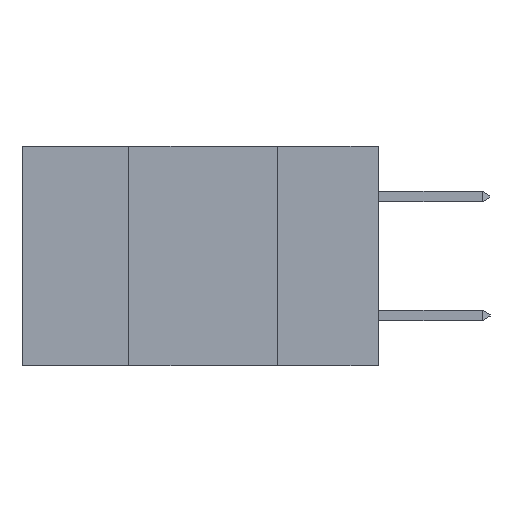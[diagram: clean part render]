
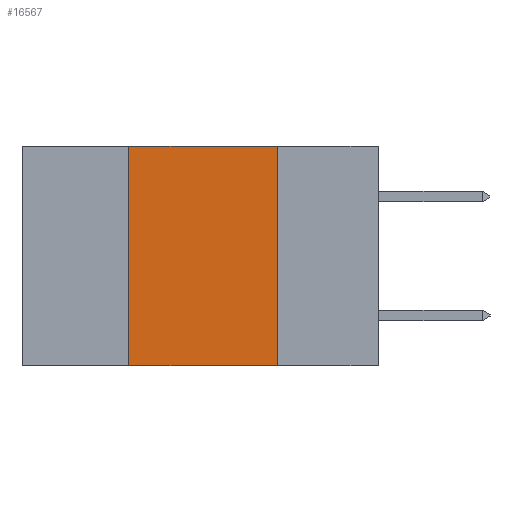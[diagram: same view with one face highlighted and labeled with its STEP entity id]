
A CAD part, left-side view. The second image highlights one B-rep face of the part: STEP entity #16567.
In plain terms, the highlighted planar face has unit normal (-1, 0, 0).
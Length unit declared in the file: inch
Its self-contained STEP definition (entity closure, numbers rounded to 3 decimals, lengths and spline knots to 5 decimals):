
#3025 = AXIS2_PLACEMENT_3D ( 'NONE', #11311, #7269, #16801 ) ;
#3606 = ORIENTED_EDGE ( 'NONE', *, *, #10193, .F. ) ;
#3710 = VERTEX_POINT ( 'NONE', #5674 ) ;
#4558 = ORIENTED_EDGE ( 'NONE', *, *, #13758, .F. ) ;
#4705 = VECTOR ( 'NONE', #7271, 39.37008 ) ;
#5646 = ORIENTED_EDGE ( 'NONE', *, *, #12043, .F. ) ;
#5674 = CARTESIAN_POINT ( 'NONE',  ( 0., 0.42, 0. ) ) ;
#5889 = PLANE ( 'NONE',  #3025 ) ;
#5892 = CARTESIAN_POINT ( 'NONE',  ( 0., 0.6, -0.37 ) ) ;
#5951 = DIRECTION ( 'NONE',  ( 0., 0., 1. ) ) ;
#6110 = VERTEX_POINT ( 'NONE', #15545 ) ;
#6960 = EDGE_CURVE ( 'NONE', #16148, #6110, #11535, .T. ) ;
#7269 = DIRECTION ( 'NONE',  ( 1., 0., 0. ) ) ;
#7271 = DIRECTION ( 'NONE',  ( 0., -1., 0. ) ) ;
#7850 = VECTOR ( 'NONE', #5951, 39.37008 ) ;
#8802 = ORIENTED_EDGE ( 'NONE', *, *, #6960, .T. ) ;
#9168 = VECTOR ( 'NONE', #14191, 39.37008 ) ;
#9660 = CARTESIAN_POINT ( 'NONE',  ( 0., 0.17, -0.37 ) ) ;
#10142 = VECTOR ( 'NONE', #11029, 39.37008 ) ;
#10193 = EDGE_CURVE ( 'NONE', #3710, #16544, #16433, .T. ) ;
#10581 = LINE ( 'NONE', #9660, #10142 ) ;
#10921 = EDGE_LOOP ( 'NONE', ( #4558, #3606, #5646, #8802 ) ) ;
#11029 = DIRECTION ( 'NONE',  ( 0., 0., -1. ) ) ;
#11311 = CARTESIAN_POINT ( 'NONE',  ( 0., 0.6, 0. ) ) ;
#11384 = CARTESIAN_POINT ( 'NONE',  ( 0., 0.42, -0.37 ) ) ;
#11535 = LINE ( 'NONE', #5892, #4705 ) ;
#11990 = CARTESIAN_POINT ( 'NONE',  ( 0., 0.42, -0.37 ) ) ;
#12043 = EDGE_CURVE ( 'NONE', #16148, #3710, #12318, .T. ) ;
#12318 = LINE ( 'NONE', #11384, #7850 ) ;
#12621 = CARTESIAN_POINT ( 'NONE',  ( 0., 0.17, 0. ) ) ;
#12800 = CARTESIAN_POINT ( 'NONE',  ( 0., 0.6, 0. ) ) ;
#13758 = EDGE_CURVE ( 'NONE', #16544, #6110, #10581, .T. ) ;
#14191 = DIRECTION ( 'NONE',  ( 0., -1., 0. ) ) ;
#15298 = FACE_OUTER_BOUND ( 'NONE', #10921, .T. ) ;
#15545 = CARTESIAN_POINT ( 'NONE',  ( 0., 0.17, -0.37 ) ) ;
#16148 = VERTEX_POINT ( 'NONE', #11990 ) ;
#16433 = LINE ( 'NONE', #12800, #9168 ) ;
#16544 = VERTEX_POINT ( 'NONE', #12621 ) ;
#16567 = ADVANCED_FACE ( 'NONE', ( #15298 ), #5889, .F. ) ;
#16801 = DIRECTION ( 'NONE',  ( 0., 0., -1. ) ) ;
